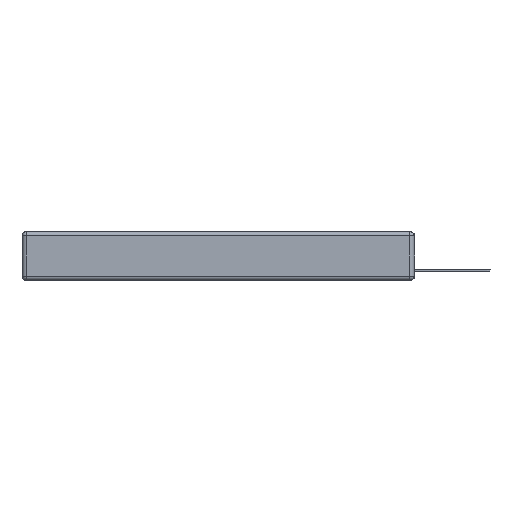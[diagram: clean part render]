
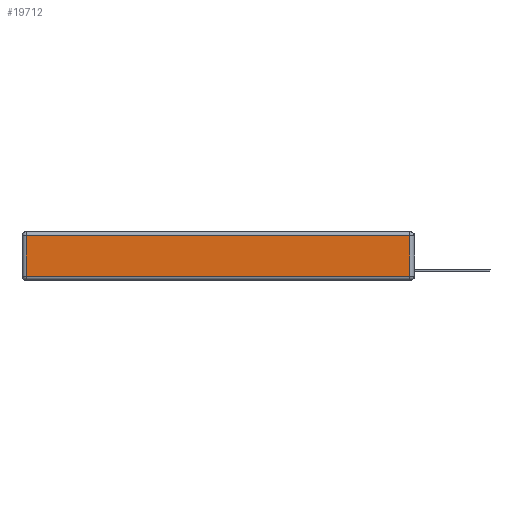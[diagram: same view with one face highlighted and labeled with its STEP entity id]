
A CAD part, left-side view. The second image highlights one B-rep face of the part: STEP entity #19712.
In plain terms, the highlighted planar face has unit normal (-1, 0, 0).
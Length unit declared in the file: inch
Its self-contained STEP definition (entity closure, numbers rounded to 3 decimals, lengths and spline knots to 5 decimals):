
#1067 = ORIENTED_EDGE ( 'NONE', *, *, #4151, .T. ) ;
#1155 = AXIS2_PLACEMENT_3D ( 'NONE', #16768, #11686, #8613 ) ;
#1880 = PLANE ( 'NONE',  #1155 ) ;
#2777 = ORIENTED_EDGE ( 'NONE', *, *, #20322, .T. ) ;
#3153 = DIRECTION ( 'NONE',  ( 0., 1., 0. ) ) ;
#3301 = CARTESIAN_POINT ( 'NONE',  ( 0., 2.72, -0.313 ) ) ;
#3550 = DIRECTION ( 'NONE',  ( 0., -1., 0. ) ) ;
#4130 = VERTEX_POINT ( 'NONE', #11261 ) ;
#4151 = EDGE_CURVE ( 'NONE', #4130, #6930, #17493, .T. ) ;
#5623 = CARTESIAN_POINT ( 'NONE',  ( 0., 0.03, -0.313 ) ) ;
#5782 = VECTOR ( 'NONE', #3550, 39.37008 ) ;
#6930 = VERTEX_POINT ( 'NONE', #12025 ) ;
#7213 = ORIENTED_EDGE ( 'NONE', *, *, #10395, .T. ) ;
#7272 = EDGE_CURVE ( 'NONE', #12084, #12977, #11427, .T. ) ;
#8613 = DIRECTION ( 'NONE',  ( 0., 0., 1. ) ) ;
#10225 = CARTESIAN_POINT ( 'NONE',  ( 0., 0., -0.313 ) ) ;
#10395 = EDGE_CURVE ( 'NONE', #12977, #4130, #11820, .T. ) ;
#11261 = CARTESIAN_POINT ( 'NONE',  ( 0., 0.03, -0.03 ) ) ;
#11427 = LINE ( 'NONE', #10225, #5782 ) ;
#11642 = LINE ( 'NONE', #13135, #16691 ) ;
#11686 = DIRECTION ( 'NONE',  ( -1., 0., 0. ) ) ;
#11820 = LINE ( 'NONE', #16699, #19899 ) ;
#12025 = CARTESIAN_POINT ( 'NONE',  ( 0., 2.72, -0.03 ) ) ;
#12084 = VERTEX_POINT ( 'NONE', #3301 ) ;
#12977 = VERTEX_POINT ( 'NONE', #5623 ) ;
#13135 = CARTESIAN_POINT ( 'NONE',  ( 0., 2.72, -0.343 ) ) ;
#13177 = VECTOR ( 'NONE', #3153, 39.37008 ) ;
#13210 = FACE_OUTER_BOUND ( 'NONE', #20010, .T. ) ;
#16156 = CARTESIAN_POINT ( 'NONE',  ( 0., 2.75, -0.03 ) ) ;
#16277 = DIRECTION ( 'NONE',  ( 0., 0., -1. ) ) ;
#16691 = VECTOR ( 'NONE', #16277, 39.37008 ) ;
#16699 = CARTESIAN_POINT ( 'NONE',  ( 0., 0.03, -0.343 ) ) ;
#16768 = CARTESIAN_POINT ( 'NONE',  ( 0., 0., -0.343 ) ) ;
#17493 = LINE ( 'NONE', #16156, #13177 ) ;
#18374 = ORIENTED_EDGE ( 'NONE', *, *, #7272, .T. ) ;
#19712 = ADVANCED_FACE ( 'NONE', ( #13210 ), #1880, .T. ) ;
#19899 = VECTOR ( 'NONE', #19954, 39.37008 ) ;
#19954 = DIRECTION ( 'NONE',  ( 0., 0., 1. ) ) ;
#20010 = EDGE_LOOP ( 'NONE', ( #18374, #7213, #1067, #2777 ) ) ;
#20322 = EDGE_CURVE ( 'NONE', #6930, #12084, #11642, .T. ) ;
